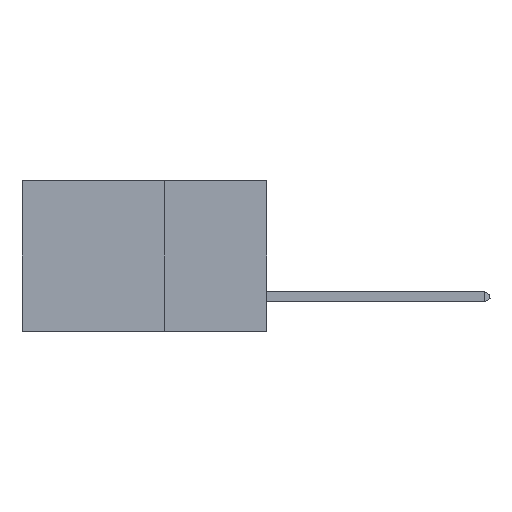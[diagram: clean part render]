
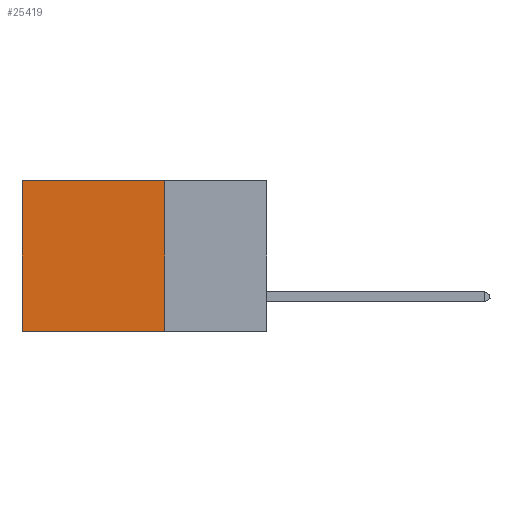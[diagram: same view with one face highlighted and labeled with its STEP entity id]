
A CAD part, left-side view. The second image highlights one B-rep face of the part: STEP entity #25419.
In plain terms, the highlighted planar face has unit normal (-1, 0, 0).
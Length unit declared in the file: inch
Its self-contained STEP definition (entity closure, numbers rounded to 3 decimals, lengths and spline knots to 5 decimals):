
#405 = LINE ( 'NONE', #2058, #13439 ) ;
#460 = PLANE ( 'NONE',  #17365 ) ;
#561 = DIRECTION ( 'NONE',  ( 0., 0., -1. ) ) ;
#756 = VECTOR ( 'NONE', #12242, 39.37008 ) ;
#802 = EDGE_CURVE ( 'NONE', #29317, #24565, #16311, .T. ) ;
#1890 = CARTESIAN_POINT ( 'NONE',  ( 0.2875, 0.25, -0.37 ) ) ;
#2058 = CARTESIAN_POINT ( 'NONE',  ( 0.2875, 0.25, 0. ) ) ;
#2185 = CARTESIAN_POINT ( 'NONE',  ( 0.2875, 0.25, 0. ) ) ;
#2882 = DIRECTION ( 'NONE',  ( 1., 0., 0. ) ) ;
#3171 = CARTESIAN_POINT ( 'NONE',  ( 0.2875, 0.6, 0. ) ) ;
#4485 = ORIENTED_EDGE ( 'NONE', *, *, #10022, .T. ) ;
#5837 = FACE_OUTER_BOUND ( 'NONE', #9893, .T. ) ;
#6047 = EDGE_CURVE ( 'NONE', #29317, #13797, #405, .T. ) ;
#6315 = ORIENTED_EDGE ( 'NONE', *, *, #6047, .F. ) ;
#9824 = CARTESIAN_POINT ( 'NONE',  ( 0.2875, 0.25, 0. ) ) ;
#9893 = EDGE_LOOP ( 'NONE', ( #4485, #10816, #6315, #22518 ) ) ;
#9933 = VECTOR ( 'NONE', #25808, 39.37008 ) ;
#10022 = EDGE_CURVE ( 'NONE', #24565, #24314, #18798, .T. ) ;
#10816 = ORIENTED_EDGE ( 'NONE', *, *, #22731, .F. ) ;
#12242 = DIRECTION ( 'NONE',  ( 0., 0., -1. ) ) ;
#13439 = VECTOR ( 'NONE', #18268, 39.37008 ) ;
#13797 = VERTEX_POINT ( 'NONE', #1890 ) ;
#15915 = CARTESIAN_POINT ( 'NONE',  ( 0.2875, 0.6, 0. ) ) ;
#16311 = LINE ( 'NONE', #26713, #26373 ) ;
#17365 = AXIS2_PLACEMENT_3D ( 'NONE', #9824, #2882, #561 ) ;
#18268 = DIRECTION ( 'NONE',  ( 0., 0., -1. ) ) ;
#18798 = LINE ( 'NONE', #3171, #756 ) ;
#22518 = ORIENTED_EDGE ( 'NONE', *, *, #802, .T. ) ;
#22731 = EDGE_CURVE ( 'NONE', #13797, #24314, #29736, .T. ) ;
#24314 = VERTEX_POINT ( 'NONE', #28100 ) ;
#24565 = VERTEX_POINT ( 'NONE', #15915 ) ;
#25157 = CARTESIAN_POINT ( 'NONE',  ( 0.2875, 0.25, -0.37 ) ) ;
#25419 = ADVANCED_FACE ( 'NONE', ( #5837 ), #460, .F. ) ;
#25808 = DIRECTION ( 'NONE',  ( 0., 1., 0. ) ) ;
#26373 = VECTOR ( 'NONE', #26410, 39.37008 ) ;
#26410 = DIRECTION ( 'NONE',  ( 0., 1., 0. ) ) ;
#26713 = CARTESIAN_POINT ( 'NONE',  ( 0.2875, 0.25, 0. ) ) ;
#28100 = CARTESIAN_POINT ( 'NONE',  ( 0.2875, 0.6, -0.37 ) ) ;
#29317 = VERTEX_POINT ( 'NONE', #2185 ) ;
#29736 = LINE ( 'NONE', #25157, #9933 ) ;
